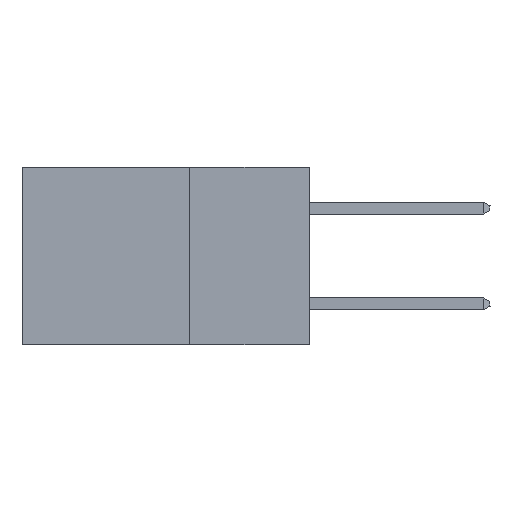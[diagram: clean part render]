
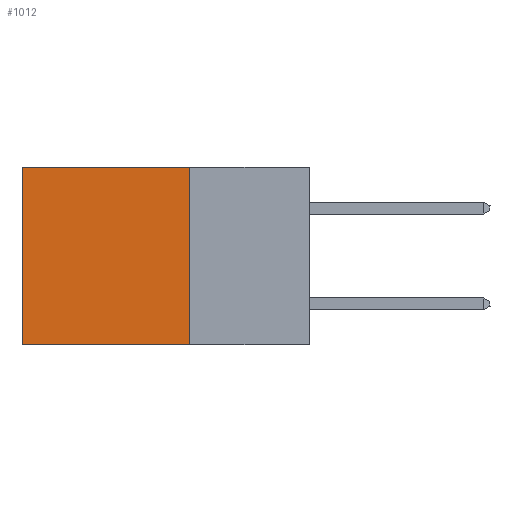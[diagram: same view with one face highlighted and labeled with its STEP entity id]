
A CAD part, left-side view. The second image highlights one B-rep face of the part: STEP entity #1012.
In plain terms, the highlighted planar face has unit normal (-1, 0, 0).
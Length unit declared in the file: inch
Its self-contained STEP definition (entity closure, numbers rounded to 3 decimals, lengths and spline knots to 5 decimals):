
#1012 = ADVANCED_FACE ( 'NONE', ( #31816 ), #2610, .F. ) ;
#1133 = CARTESIAN_POINT ( 'NONE',  ( 0.2875, 0.6, 0. ) ) ;
#2610 = PLANE ( 'NONE',  #38802 ) ;
#4910 = ORIENTED_EDGE ( 'NONE', *, *, #11591, .F. ) ;
#5538 = VECTOR ( 'NONE', #8878, 39.37008 ) ;
#7809 = EDGE_CURVE ( 'NONE', #25617, #27866, #9004, .T. ) ;
#8599 = CARTESIAN_POINT ( 'NONE',  ( 0.2875, 0.25, 0. ) ) ;
#8878 = DIRECTION ( 'NONE',  ( 0., 1., 0. ) ) ;
#9004 = LINE ( 'NONE', #27797, #34657 ) ;
#9511 = VERTEX_POINT ( 'NONE', #31492 ) ;
#11475 = LINE ( 'NONE', #32010, #33802 ) ;
#11591 = EDGE_CURVE ( 'NONE', #28734, #9511, #26084, .T. ) ;
#13237 = DIRECTION ( 'NONE',  ( 0., 0., -1. ) ) ;
#13393 = EDGE_CURVE ( 'NONE', #25617, #28734, #36798, .T. ) ;
#17430 = EDGE_LOOP ( 'NONE', ( #19390, #4910, #29245, #39344 ) ) ;
#17646 = DIRECTION ( 'NONE',  ( 0., 0., -1. ) ) ;
#19390 = ORIENTED_EDGE ( 'NONE', *, *, #22253, .T. ) ;
#19775 = DIRECTION ( 'NONE',  ( 0., 1., 0. ) ) ;
#19892 = CARTESIAN_POINT ( 'NONE',  ( 0.2875, 0.25, -0.37 ) ) ;
#22253 = EDGE_CURVE ( 'NONE', #27866, #9511, #11475, .T. ) ;
#25617 = VERTEX_POINT ( 'NONE', #29327 ) ;
#26084 = LINE ( 'NONE', #36364, #5538 ) ;
#27797 = CARTESIAN_POINT ( 'NONE',  ( 0.2875, 0.25, 0. ) ) ;
#27866 = VERTEX_POINT ( 'NONE', #1133 ) ;
#28734 = VERTEX_POINT ( 'NONE', #19892 ) ;
#29245 = ORIENTED_EDGE ( 'NONE', *, *, #13393, .F. ) ;
#29327 = CARTESIAN_POINT ( 'NONE',  ( 0.2875, 0.25, 0. ) ) ;
#29333 = VECTOR ( 'NONE', #39284, 39.37008 ) ;
#31492 = CARTESIAN_POINT ( 'NONE',  ( 0.2875, 0.6, -0.37 ) ) ;
#31816 = FACE_OUTER_BOUND ( 'NONE', #17430, .T. ) ;
#32010 = CARTESIAN_POINT ( 'NONE',  ( 0.2875, 0.6, 0. ) ) ;
#32676 = DIRECTION ( 'NONE',  ( 1., 0., 0. ) ) ;
#33802 = VECTOR ( 'NONE', #13237, 39.37008 ) ;
#34657 = VECTOR ( 'NONE', #19775, 39.37008 ) ;
#35582 = CARTESIAN_POINT ( 'NONE',  ( 0.2875, 0.25, 0. ) ) ;
#36364 = CARTESIAN_POINT ( 'NONE',  ( 0.2875, 0.25, -0.37 ) ) ;
#36798 = LINE ( 'NONE', #8599, #29333 ) ;
#38802 = AXIS2_PLACEMENT_3D ( 'NONE', #35582, #32676, #17646 ) ;
#39284 = DIRECTION ( 'NONE',  ( 0., 0., -1. ) ) ;
#39344 = ORIENTED_EDGE ( 'NONE', *, *, #7809, .T. ) ;
